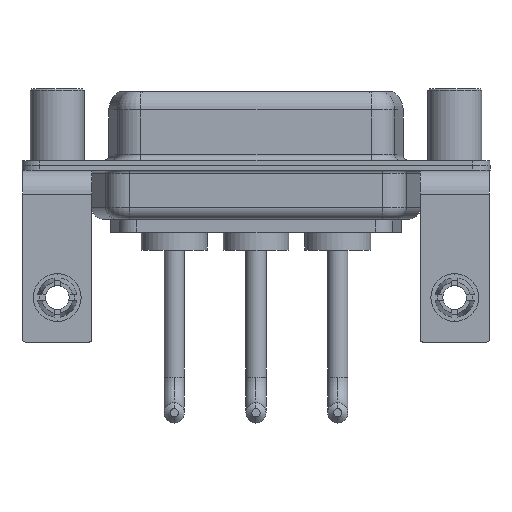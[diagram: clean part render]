
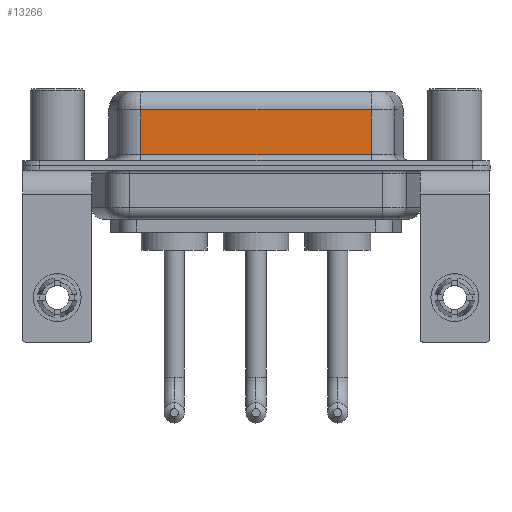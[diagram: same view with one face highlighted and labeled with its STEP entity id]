
A CAD part, front view. The second image highlights one B-rep face of the part: STEP entity #13266.
In plain terms, the highlighted planar face has unit normal (0, -1, 0).
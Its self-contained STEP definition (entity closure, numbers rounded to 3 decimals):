
#597 = CARTESIAN_POINT ( 'NONE',  ( 7.013, -3.95, 0.9 ) ) ;
#642 = LINE ( 'NONE', #6998, #3341 ) ;
#788 = ORIENTED_EDGE ( 'NONE', *, *, #9057, .T. ) ;
#994 = DIRECTION ( 'NONE',  ( 0., 1., 0. ) ) ;
#1938 = CARTESIAN_POINT ( 'NONE',  ( 26.287, -3.95, 6.4 ) ) ;
#2553 = EDGE_CURVE ( 'NONE', #13320, #8639, #6675, .T. ) ;
#2648 = CARTESIAN_POINT ( 'NONE',  ( 26.287, -3.95, 0.9 ) ) ;
#3177 = VECTOR ( 'NONE', #7844, 1000. ) ;
#3341 = VECTOR ( 'NONE', #11846, 1000. ) ;
#4148 = DIRECTION ( 'NONE',  ( 1., 0., 0. ) ) ;
#4228 = LINE ( 'NONE', #2648, #11772 ) ;
#4266 = DIRECTION ( 'NONE',  ( 0., 0., 1. ) ) ;
#4507 = ORIENTED_EDGE ( 'NONE', *, *, #5636, .T. ) ;
#5632 = VECTOR ( 'NONE', #9338, 1000. ) ;
#5636 = EDGE_CURVE ( 'NONE', #8639, #13302, #8006, .T. ) ;
#5977 = VERTEX_POINT ( 'NONE', #15390 ) ;
#6675 = LINE ( 'NONE', #13101, #5632 ) ;
#6998 = CARTESIAN_POINT ( 'NONE',  ( 26.287, -3.95, 6.4 ) ) ;
#7094 = AXIS2_PLACEMENT_3D ( 'NONE', #1938, #994, #4266 ) ;
#7474 = ORIENTED_EDGE ( 'NONE', *, *, #2553, .T. ) ;
#7636 = FACE_OUTER_BOUND ( 'NONE', #14054, .T. ) ;
#7844 = DIRECTION ( 'NONE',  ( 0., 0., -1. ) ) ;
#7852 = CARTESIAN_POINT ( 'NONE',  ( 7.013, -3.95, 4.65 ) ) ;
#8006 = LINE ( 'NONE', #14262, #3177 ) ;
#8595 = PLANE ( 'NONE',  #7094 ) ;
#8639 = VERTEX_POINT ( 'NONE', #7852 ) ;
#9057 = EDGE_CURVE ( 'NONE', #13302, #5977, #4228, .T. ) ;
#9338 = DIRECTION ( 'NONE',  ( -1., 0., 0. ) ) ;
#9526 = ORIENTED_EDGE ( 'NONE', *, *, #15399, .F. ) ;
#11772 = VECTOR ( 'NONE', #4148, 1000. ) ;
#11846 = DIRECTION ( 'NONE',  ( 0., 0., -1. ) ) ;
#13101 = CARTESIAN_POINT ( 'NONE',  ( 26.287, -3.95, 4.65 ) ) ;
#13266 = ADVANCED_FACE ( 'NONE', ( #7636 ), #8595, .F. ) ;
#13302 = VERTEX_POINT ( 'NONE', #597 ) ;
#13320 = VERTEX_POINT ( 'NONE', #14939 ) ;
#14054 = EDGE_LOOP ( 'NONE', ( #9526, #7474, #4507, #788 ) ) ;
#14262 = CARTESIAN_POINT ( 'NONE',  ( 7.013, -3.95, 6.4 ) ) ;
#14939 = CARTESIAN_POINT ( 'NONE',  ( 26.287, -3.95, 4.65 ) ) ;
#15390 = CARTESIAN_POINT ( 'NONE',  ( 26.287, -3.95, 0.9 ) ) ;
#15399 = EDGE_CURVE ( 'NONE', #13320, #5977, #642, .T. ) ;
